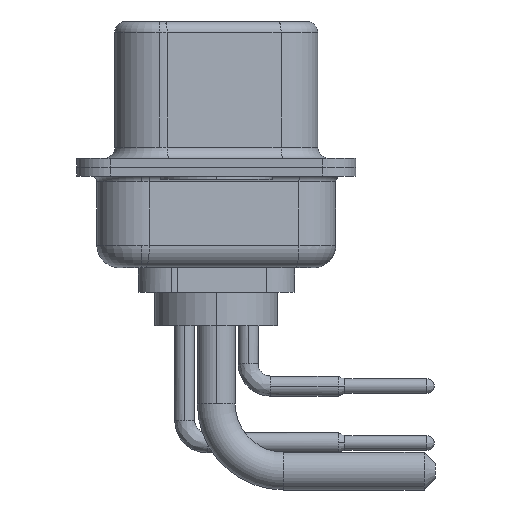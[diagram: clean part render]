
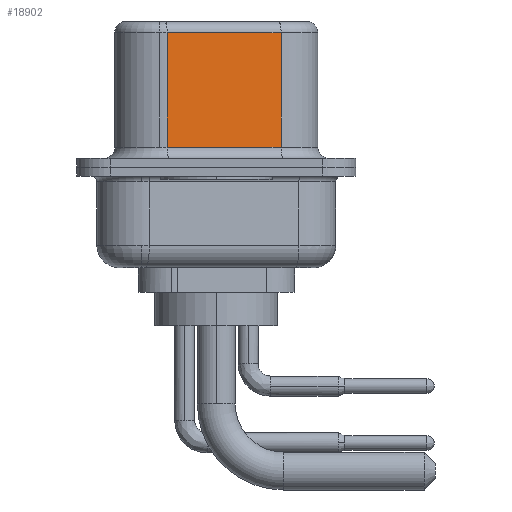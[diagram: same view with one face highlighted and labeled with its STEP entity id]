
A CAD part, left-side view. The second image highlights one B-rep face of the part: STEP entity #18902.
In plain terms, the highlighted planar face has unit normal (-0.985, -0.174, 0).
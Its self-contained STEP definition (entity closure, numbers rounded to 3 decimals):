
#94 = PLANE ( 'NONE',  #14676 ) ;
#1183 = CARTESIAN_POINT ( 'NONE',  ( 4.58, -2.897, 0.9 ) ) ;
#1749 = FACE_OUTER_BOUND ( 'NONE', #5447, .T. ) ;
#2106 = LINE ( 'NONE', #15663, #8337 ) ;
#2114 = EDGE_CURVE ( 'NONE', #9316, #16611, #13054, .T. ) ;
#2398 = LINE ( 'NONE', #9441, #13034 ) ;
#3216 = EDGE_CURVE ( 'NONE', #16614, #18340, #2106, .T. ) ;
#4048 = DIRECTION ( 'NONE',  ( -0.174, 0.985, 0. ) ) ;
#5447 = EDGE_LOOP ( 'NONE', ( #12960, #7451, #16033, #8090 ) ) ;
#7451 = ORIENTED_EDGE ( 'NONE', *, *, #19170, .T. ) ;
#8090 = ORIENTED_EDGE ( 'NONE', *, *, #9164, .T. ) ;
#8337 = VECTOR ( 'NONE', #22760, 1000. ) ;
#9164 = EDGE_CURVE ( 'NONE', #16611, #18340, #2398, .T. ) ;
#9316 = VERTEX_POINT ( 'NONE', #10019 ) ;
#9441 = CARTESIAN_POINT ( 'NONE',  ( 4.58, -2.897, 0.9 ) ) ;
#9840 = VECTOR ( 'NONE', #12935, 1000. ) ;
#9931 = CARTESIAN_POINT ( 'NONE',  ( 3.68, 2.203, 6.52 ) ) ;
#10019 = CARTESIAN_POINT ( 'NONE',  ( 3.68, 2.203, 6.02 ) ) ;
#10525 = DIRECTION ( 'NONE',  ( -0.174, 0.985, 0. ) ) ;
#11327 = LINE ( 'NONE', #13189, #15797 ) ;
#12252 = DIRECTION ( 'NONE',  ( 0.985, 0.174, 0. ) ) ;
#12626 = CARTESIAN_POINT ( 'NONE',  ( 3.68, 2.203, 0.9 ) ) ;
#12935 = DIRECTION ( 'NONE',  ( 0., 0., -1. ) ) ;
#12960 = ORIENTED_EDGE ( 'NONE', *, *, #3216, .F. ) ;
#13034 = VECTOR ( 'NONE', #18511, 1000. ) ;
#13054 = LINE ( 'NONE', #9931, #9840 ) ;
#13189 = CARTESIAN_POINT ( 'NONE',  ( 4.58, -2.897, 6.02 ) ) ;
#13936 = CARTESIAN_POINT ( 'NONE',  ( 4.58, -2.897, 6.02 ) ) ;
#14232 = CARTESIAN_POINT ( 'NONE',  ( 4.58, -2.897, 6.52 ) ) ;
#14676 = AXIS2_PLACEMENT_3D ( 'NONE', #14232, #12252, #10525 ) ;
#15663 = CARTESIAN_POINT ( 'NONE',  ( 4.58, -2.897, 6.52 ) ) ;
#15797 = VECTOR ( 'NONE', #4048, 1000. ) ;
#16033 = ORIENTED_EDGE ( 'NONE', *, *, #2114, .T. ) ;
#16611 = VERTEX_POINT ( 'NONE', #12626 ) ;
#16614 = VERTEX_POINT ( 'NONE', #13936 ) ;
#18340 = VERTEX_POINT ( 'NONE', #1183 ) ;
#18511 = DIRECTION ( 'NONE',  ( 0.174, -0.985, 0. ) ) ;
#18902 = ADVANCED_FACE ( 'NONE', ( #1749 ), #94, .F. ) ;
#19170 = EDGE_CURVE ( 'NONE', #16614, #9316, #11327, .T. ) ;
#22760 = DIRECTION ( 'NONE',  ( 0., 0., -1. ) ) ;
